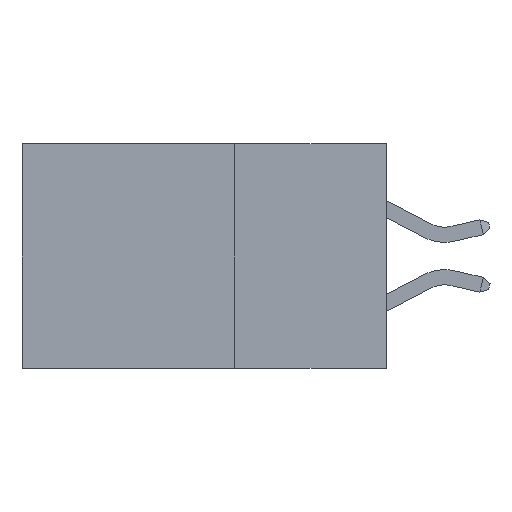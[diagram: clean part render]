
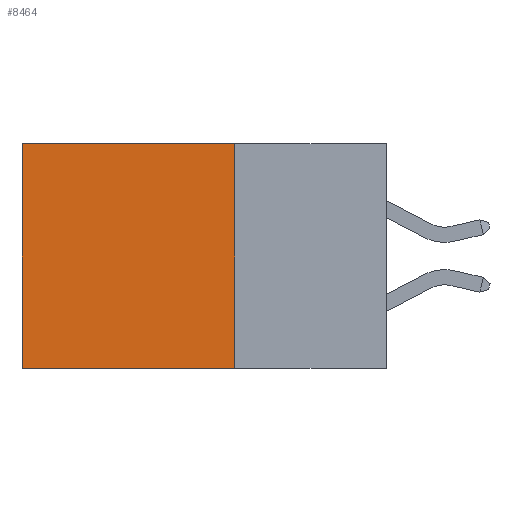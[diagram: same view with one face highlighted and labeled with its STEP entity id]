
A CAD part, left-side view. The second image highlights one B-rep face of the part: STEP entity #8464.
In plain terms, the highlighted planar face has unit normal (-1, 0, 0).
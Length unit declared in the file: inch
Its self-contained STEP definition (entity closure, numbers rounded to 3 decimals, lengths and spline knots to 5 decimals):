
#139 = EDGE_CURVE ( 'NONE', #1771, #4878, #1467, .T. ) ;
#523 = CARTESIAN_POINT ( 'NONE',  ( 0.2615, 0.6, -0.37 ) ) ;
#1184 = FACE_OUTER_BOUND ( 'NONE', #8698, .T. ) ;
#1467 = LINE ( 'NONE', #5160, #17760 ) ;
#1771 = VERTEX_POINT ( 'NONE', #24713 ) ;
#2140 = CARTESIAN_POINT ( 'NONE',  ( 0.2615, 0.6, -0.37 ) ) ;
#2495 = EDGE_CURVE ( 'NONE', #4878, #13344, #24524, .T. ) ;
#3699 = VERTEX_POINT ( 'NONE', #17767 ) ;
#4760 = ORIENTED_EDGE ( 'NONE', *, *, #139, .F. ) ;
#4878 = VERTEX_POINT ( 'NONE', #20821 ) ;
#5160 = CARTESIAN_POINT ( 'NONE',  ( 0.2615, 0.25, -0.37 ) ) ;
#6853 = DIRECTION ( 'NONE',  ( 0., 0., -1. ) ) ;
#8247 = CARTESIAN_POINT ( 'NONE',  ( 0.2615, 0.25, -0.37 ) ) ;
#8464 = ADVANCED_FACE ( 'NONE', ( #1184 ), #12171, .F. ) ;
#8698 = EDGE_LOOP ( 'NONE', ( #16955, #12484, #4760, #13600 ) ) ;
#9777 = EDGE_CURVE ( 'NONE', #3699, #13344, #24616, .T. ) ;
#10289 = DIRECTION ( 'NONE',  ( 0., 0., -1. ) ) ;
#10564 = LINE ( 'NONE', #13366, #25339 ) ;
#12171 = PLANE ( 'NONE',  #22992 ) ;
#12484 = ORIENTED_EDGE ( 'NONE', *, *, #2495, .F. ) ;
#13301 = VECTOR ( 'NONE', #18481, 39.37008 ) ;
#13344 = VERTEX_POINT ( 'NONE', #523 ) ;
#13366 = CARTESIAN_POINT ( 'NONE',  ( 0.2615, 0.25, 0. ) ) ;
#13600 = ORIENTED_EDGE ( 'NONE', *, *, #20997, .T. ) ;
#14693 = DIRECTION ( 'NONE',  ( 0., 1., 0. ) ) ;
#16955 = ORIENTED_EDGE ( 'NONE', *, *, #9777, .T. ) ;
#17760 = VECTOR ( 'NONE', #6853, 39.37008 ) ;
#17767 = CARTESIAN_POINT ( 'NONE',  ( 0.2615, 0.6, 0. ) ) ;
#18481 = DIRECTION ( 'NONE',  ( 0., 0., -1. ) ) ;
#19211 = VECTOR ( 'NONE', #14693, 39.37008 ) ;
#20760 = CARTESIAN_POINT ( 'NONE',  ( 0.2615, 0.25, -0.37 ) ) ;
#20821 = CARTESIAN_POINT ( 'NONE',  ( 0.2615, 0.25, -0.37 ) ) ;
#20997 = EDGE_CURVE ( 'NONE', #1771, #3699, #10564, .T. ) ;
#22394 = DIRECTION ( 'NONE',  ( 1., 0., 0. ) ) ;
#22992 = AXIS2_PLACEMENT_3D ( 'NONE', #8247, #22394, #10289 ) ;
#23492 = DIRECTION ( 'NONE',  ( 0., 1., 0. ) ) ;
#24524 = LINE ( 'NONE', #20760, #19211 ) ;
#24616 = LINE ( 'NONE', #2140, #13301 ) ;
#24713 = CARTESIAN_POINT ( 'NONE',  ( 0.2615, 0.25, 0. ) ) ;
#25339 = VECTOR ( 'NONE', #23492, 39.37008 ) ;
